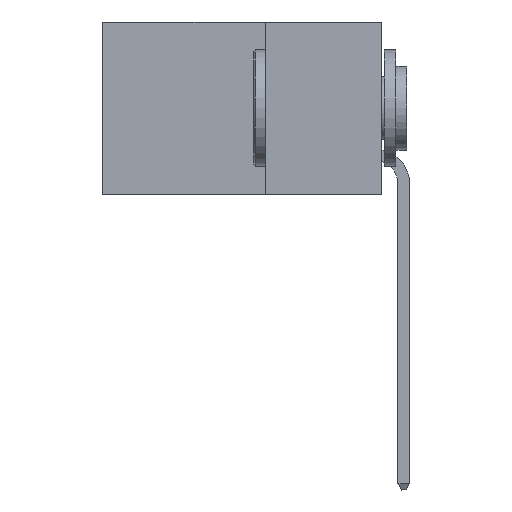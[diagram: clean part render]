
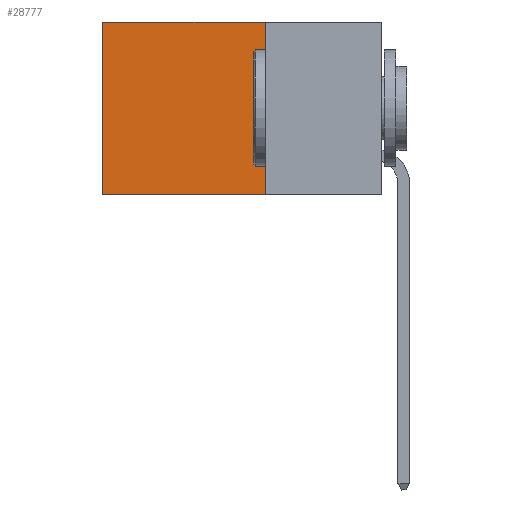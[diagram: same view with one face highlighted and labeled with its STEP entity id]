
A CAD part, left-side view. The second image highlights one B-rep face of the part: STEP entity #28777.
In plain terms, the highlighted planar face has unit normal (-1, 0, 0).
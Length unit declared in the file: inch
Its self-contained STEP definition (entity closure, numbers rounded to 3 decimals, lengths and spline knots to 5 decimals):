
#632 = VECTOR ( 'NONE', #28493, 39.37008 ) ;
#2562 = CARTESIAN_POINT ( 'NONE',  ( 0.2875, 0.6, 0. ) ) ;
#2937 = PLANE ( 'NONE',  #32604 ) ;
#4138 = EDGE_CURVE ( 'NONE', #33689, #17938, #25851, .T. ) ;
#4217 = DIRECTION ( 'NONE',  ( 0., 0., -1. ) ) ;
#9807 = VECTOR ( 'NONE', #4217, 39.37008 ) ;
#10337 = CARTESIAN_POINT ( 'NONE',  ( 0.2875, 0.25, -0.37 ) ) ;
#12552 = CARTESIAN_POINT ( 'NONE',  ( 0.2875, 0.6, 0. ) ) ;
#12566 = CARTESIAN_POINT ( 'NONE',  ( 0.2875, 0.25, 0. ) ) ;
#17283 = DIRECTION ( 'NONE',  ( 0., 1., 0. ) ) ;
#17565 = VECTOR ( 'NONE', #17283, 39.37008 ) ;
#17938 = VERTEX_POINT ( 'NONE', #2562 ) ;
#18509 = ORIENTED_EDGE ( 'NONE', *, *, #4138, .T. ) ;
#18708 = EDGE_LOOP ( 'NONE', ( #32471, #28550, #20879, #18509 ) ) ;
#20879 = ORIENTED_EDGE ( 'NONE', *, *, #22562, .F. ) ;
#21362 = DIRECTION ( 'NONE',  ( 0., 1., 0. ) ) ;
#21918 = EDGE_CURVE ( 'NONE', #25620, #39533, #33853, .T. ) ;
#22562 = EDGE_CURVE ( 'NONE', #33689, #25620, #39592, .T. ) ;
#24659 = DIRECTION ( 'NONE',  ( 1., 0., 0. ) ) ;
#25418 = CARTESIAN_POINT ( 'NONE',  ( 0.2875, 0.25, -0.37 ) ) ;
#25479 = VECTOR ( 'NONE', #21362, 39.37008 ) ;
#25620 = VERTEX_POINT ( 'NONE', #25418 ) ;
#25851 = LINE ( 'NONE', #35985, #17565 ) ;
#27580 = LINE ( 'NONE', #12552, #632 ) ;
#28493 = DIRECTION ( 'NONE',  ( 0., 0., -1. ) ) ;
#28550 = ORIENTED_EDGE ( 'NONE', *, *, #21918, .F. ) ;
#28777 = ADVANCED_FACE ( 'NONE', ( #38668 ), #2937, .F. ) ;
#32471 = ORIENTED_EDGE ( 'NONE', *, *, #35459, .T. ) ;
#32604 = AXIS2_PLACEMENT_3D ( 'NONE', #12566, #24659, #40397 ) ;
#33689 = VERTEX_POINT ( 'NONE', #38484 ) ;
#33853 = LINE ( 'NONE', #10337, #25479 ) ;
#35297 = CARTESIAN_POINT ( 'NONE',  ( 0.2875, 0.25, 0. ) ) ;
#35459 = EDGE_CURVE ( 'NONE', #17938, #39533, #27580, .T. ) ;
#35985 = CARTESIAN_POINT ( 'NONE',  ( 0.2875, 0.25, 0. ) ) ;
#38484 = CARTESIAN_POINT ( 'NONE',  ( 0.2875, 0.25, 0. ) ) ;
#38668 = FACE_OUTER_BOUND ( 'NONE', #18708, .T. ) ;
#39114 = CARTESIAN_POINT ( 'NONE',  ( 0.2875, 0.6, -0.37 ) ) ;
#39533 = VERTEX_POINT ( 'NONE', #39114 ) ;
#39592 = LINE ( 'NONE', #35297, #9807 ) ;
#40397 = DIRECTION ( 'NONE',  ( 0., 0., -1. ) ) ;
